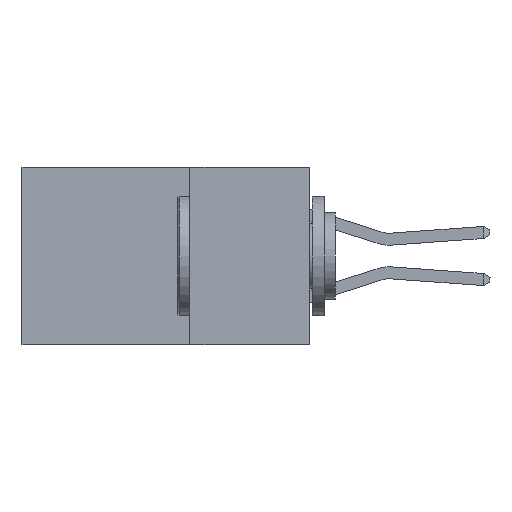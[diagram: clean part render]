
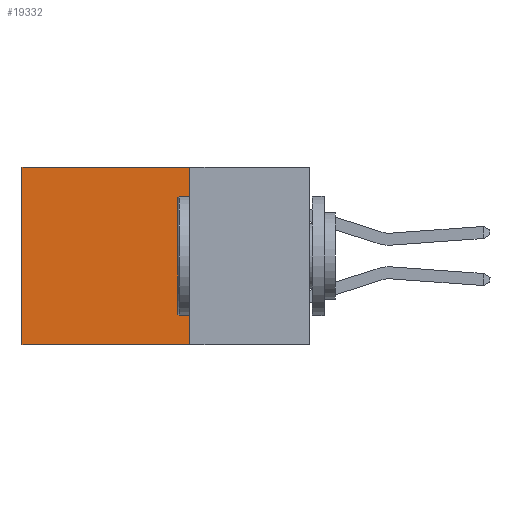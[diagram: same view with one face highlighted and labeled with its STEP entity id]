
A CAD part, left-side view. The second image highlights one B-rep face of the part: STEP entity #19332.
In plain terms, the highlighted planar face has unit normal (-1, 0, 0).
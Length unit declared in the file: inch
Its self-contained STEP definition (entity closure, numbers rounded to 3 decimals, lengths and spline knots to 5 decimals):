
#353 = ORIENTED_EDGE ( 'NONE', *, *, #13513, .F. ) ;
#419 = VERTEX_POINT ( 'NONE', #10655 ) ;
#1814 = CARTESIAN_POINT ( 'NONE',  ( 0.298, 0.25, 0. ) ) ;
#2262 = VERTEX_POINT ( 'NONE', #3907 ) ;
#2326 = ORIENTED_EDGE ( 'NONE', *, *, #11126, .T. ) ;
#2885 = AXIS2_PLACEMENT_3D ( 'NONE', #14043, #9335, #20175 ) ;
#3414 = LINE ( 'NONE', #19283, #8109 ) ;
#3503 = EDGE_CURVE ( 'NONE', #19499, #2262, #3414, .T. ) ;
#3907 = CARTESIAN_POINT ( 'NONE',  ( 0.298, 0.25, -0.37 ) ) ;
#4539 = LINE ( 'NONE', #11343, #8203 ) ;
#6144 = ORIENTED_EDGE ( 'NONE', *, *, #3503, .F. ) ;
#6259 = LINE ( 'NONE', #9063, #18200 ) ;
#8109 = VECTOR ( 'NONE', #19199, 39.37008 ) ;
#8203 = VECTOR ( 'NONE', #14537, 39.37008 ) ;
#9063 = CARTESIAN_POINT ( 'NONE',  ( 0.298, 0.6, 0. ) ) ;
#9335 = DIRECTION ( 'NONE',  ( 1., 0., 0. ) ) ;
#9352 = CARTESIAN_POINT ( 'NONE',  ( 0.298, 0.6, -0.37 ) ) ;
#10655 = CARTESIAN_POINT ( 'NONE',  ( 0.298, 0.6, 0. ) ) ;
#10828 = EDGE_CURVE ( 'NONE', #419, #10929, #6259, .T. ) ;
#10929 = VERTEX_POINT ( 'NONE', #9352 ) ;
#11126 = EDGE_CURVE ( 'NONE', #19499, #419, #4539, .T. ) ;
#11343 = CARTESIAN_POINT ( 'NONE',  ( 0.298, 0.25, 0. ) ) ;
#12436 = PLANE ( 'NONE',  #2885 ) ;
#13513 = EDGE_CURVE ( 'NONE', #2262, #10929, #14025, .T. ) ;
#13840 = DIRECTION ( 'NONE',  ( 0., 0., -1. ) ) ;
#14025 = LINE ( 'NONE', #18692, #17153 ) ;
#14043 = CARTESIAN_POINT ( 'NONE',  ( 0.298, 0.25, 0. ) ) ;
#14121 = FACE_OUTER_BOUND ( 'NONE', #14312, .T. ) ;
#14312 = EDGE_LOOP ( 'NONE', ( #17263, #353, #6144, #2326 ) ) ;
#14537 = DIRECTION ( 'NONE',  ( 0., 1., 0. ) ) ;
#17153 = VECTOR ( 'NONE', #20299, 39.37008 ) ;
#17263 = ORIENTED_EDGE ( 'NONE', *, *, #10828, .T. ) ;
#18200 = VECTOR ( 'NONE', #13840, 39.37008 ) ;
#18692 = CARTESIAN_POINT ( 'NONE',  ( 0.298, 0.25, -0.37 ) ) ;
#19199 = DIRECTION ( 'NONE',  ( 0., 0., -1. ) ) ;
#19283 = CARTESIAN_POINT ( 'NONE',  ( 0.298, 0.25, 0. ) ) ;
#19332 = ADVANCED_FACE ( 'NONE', ( #14121 ), #12436, .F. ) ;
#19499 = VERTEX_POINT ( 'NONE', #1814 ) ;
#20175 = DIRECTION ( 'NONE',  ( 0., 0., -1. ) ) ;
#20299 = DIRECTION ( 'NONE',  ( 0., 1., 0. ) ) ;
